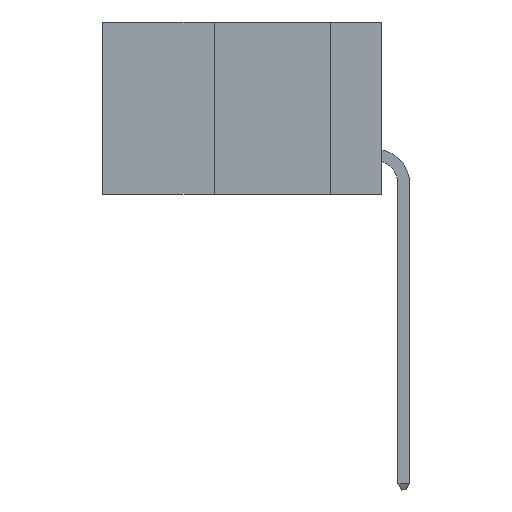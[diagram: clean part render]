
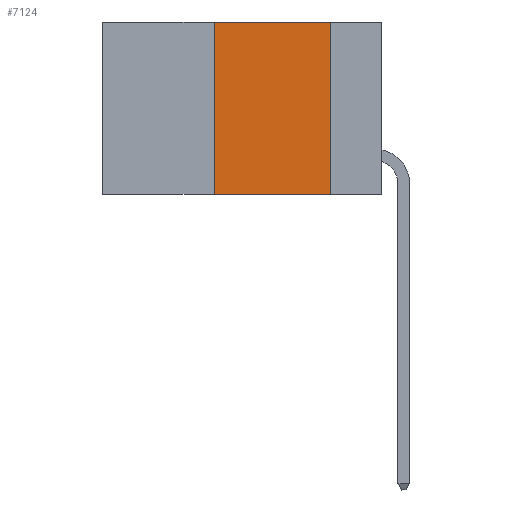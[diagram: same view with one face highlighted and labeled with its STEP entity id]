
A CAD part, left-side view. The second image highlights one B-rep face of the part: STEP entity #7124.
In plain terms, the highlighted planar face has unit normal (-1, 0, 0).
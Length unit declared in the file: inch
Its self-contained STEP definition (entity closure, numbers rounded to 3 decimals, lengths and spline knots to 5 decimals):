
#12 = LINE ( 'NONE', #5888, #7388 ) ;
#184 = ORIENTED_EDGE ( 'NONE', *, *, #11175, .F. ) ;
#881 = PLANE ( 'NONE',  #4367 ) ;
#943 = EDGE_LOOP ( 'NONE', ( #184, #4418, #10974, #3184 ) ) ;
#1030 = EDGE_CURVE ( 'NONE', #1516, #8270, #4209, .T. ) ;
#1516 = VERTEX_POINT ( 'NONE', #10009 ) ;
#1953 = DIRECTION ( 'NONE',  ( 1., 0., 0. ) ) ;
#2506 = DIRECTION ( 'NONE',  ( 0., -1., 0. ) ) ;
#3012 = CARTESIAN_POINT ( 'NONE',  ( 0., 0.6, 0. ) ) ;
#3079 = CARTESIAN_POINT ( 'NONE',  ( 0., 0.11, 0. ) ) ;
#3184 = ORIENTED_EDGE ( 'NONE', *, *, #6682, .T. ) ;
#4209 = LINE ( 'NONE', #5077, #13137 ) ;
#4367 = AXIS2_PLACEMENT_3D ( 'NONE', #3012, #1953, #13085 ) ;
#4418 = ORIENTED_EDGE ( 'NONE', *, *, #1030, .F. ) ;
#4520 = CARTESIAN_POINT ( 'NONE',  ( 0., 0.11, -0.37 ) ) ;
#5077 = CARTESIAN_POINT ( 'NONE',  ( 0., 0.6, 0. ) ) ;
#5888 = CARTESIAN_POINT ( 'NONE',  ( 0., 0.11, 0. ) ) ;
#5961 = EDGE_CURVE ( 'NONE', #6497, #1516, #9199, .T. ) ;
#5971 = CARTESIAN_POINT ( 'NONE',  ( 0., 0.36, 0. ) ) ;
#6497 = VERTEX_POINT ( 'NONE', #9383 ) ;
#6682 = EDGE_CURVE ( 'NONE', #6497, #7515, #7397, .T. ) ;
#6983 = DIRECTION ( 'NONE',  ( 0., 0., 1. ) ) ;
#7124 = ADVANCED_FACE ( 'NONE', ( #7238 ), #881, .F. ) ;
#7238 = FACE_OUTER_BOUND ( 'NONE', #943, .T. ) ;
#7388 = VECTOR ( 'NONE', #9954, 39.37008 ) ;
#7397 = LINE ( 'NONE', #10219, #11883 ) ;
#7515 = VERTEX_POINT ( 'NONE', #4520 ) ;
#8270 = VERTEX_POINT ( 'NONE', #3079 ) ;
#9199 = LINE ( 'NONE', #5971, #11427 ) ;
#9383 = CARTESIAN_POINT ( 'NONE',  ( 0., 0.36, -0.37 ) ) ;
#9954 = DIRECTION ( 'NONE',  ( 0., 0., -1. ) ) ;
#10009 = CARTESIAN_POINT ( 'NONE',  ( 0., 0.36, 0. ) ) ;
#10219 = CARTESIAN_POINT ( 'NONE',  ( 0., 0.6, -0.37 ) ) ;
#10237 = DIRECTION ( 'NONE',  ( 0., -1., 0. ) ) ;
#10974 = ORIENTED_EDGE ( 'NONE', *, *, #5961, .F. ) ;
#11175 = EDGE_CURVE ( 'NONE', #8270, #7515, #12, .T. ) ;
#11427 = VECTOR ( 'NONE', #6983, 39.37008 ) ;
#11883 = VECTOR ( 'NONE', #2506, 39.37008 ) ;
#13085 = DIRECTION ( 'NONE',  ( 0., 0., -1. ) ) ;
#13137 = VECTOR ( 'NONE', #10237, 39.37008 ) ;
